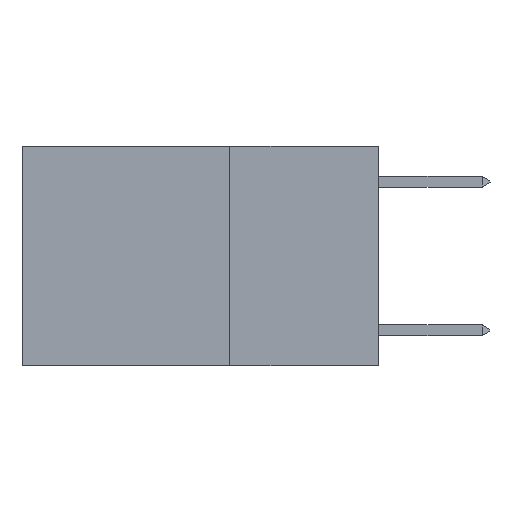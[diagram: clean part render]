
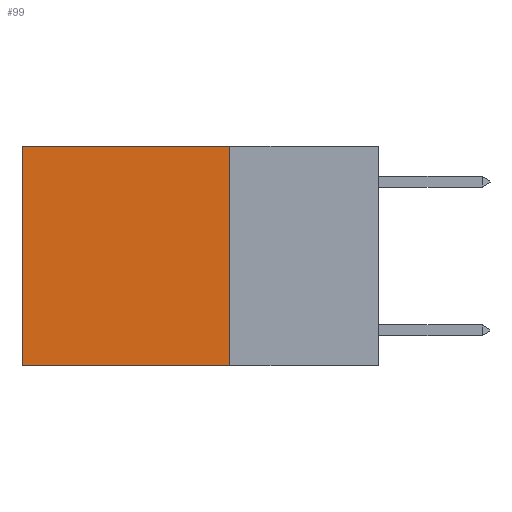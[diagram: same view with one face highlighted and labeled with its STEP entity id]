
A CAD part, left-side view. The second image highlights one B-rep face of the part: STEP entity #99.
In plain terms, the highlighted planar face has unit normal (-1, 0, 0).
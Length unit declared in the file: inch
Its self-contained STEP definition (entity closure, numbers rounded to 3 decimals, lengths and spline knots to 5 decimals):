
#99 = ADVANCED_FACE ( 'NONE', ( #2087 ), #13242, .F. ) ;
#350 = CARTESIAN_POINT ( 'NONE',  ( 0.2625, 0.25, 0. ) ) ;
#652 = CARTESIAN_POINT ( 'NONE',  ( 0.2625, 0.6, -0.37 ) ) ;
#1830 = VECTOR ( 'NONE', #3818, 39.37008 ) ;
#1869 = CARTESIAN_POINT ( 'NONE',  ( 0.2625, 0.6, 0. ) ) ;
#2087 = FACE_OUTER_BOUND ( 'NONE', #12609, .T. ) ;
#2498 = ORIENTED_EDGE ( 'NONE', *, *, #12370, .F. ) ;
#2987 = VERTEX_POINT ( 'NONE', #1869 ) ;
#3550 = CARTESIAN_POINT ( 'NONE',  ( 0.2625, 0.6, 0. ) ) ;
#3818 = DIRECTION ( 'NONE',  ( 0., 1., 0. ) ) ;
#4362 = VERTEX_POINT ( 'NONE', #11102 ) ;
#4703 = DIRECTION ( 'NONE',  ( 0., 1., 0. ) ) ;
#4792 = AXIS2_PLACEMENT_3D ( 'NONE', #12082, #13110, #10972 ) ;
#6037 = DIRECTION ( 'NONE',  ( 0., 0., -1. ) ) ;
#6548 = DIRECTION ( 'NONE',  ( 0., 0., -1. ) ) ;
#7087 = ORIENTED_EDGE ( 'NONE', *, *, #10981, .T. ) ;
#8176 = LINE ( 'NONE', #12398, #11450 ) ;
#8315 = ORIENTED_EDGE ( 'NONE', *, *, #11752, .T. ) ;
#8444 = VECTOR ( 'NONE', #6548, 39.37008 ) ;
#9269 = CARTESIAN_POINT ( 'NONE',  ( 0.2625, 0.25, -0.37 ) ) ;
#9919 = LINE ( 'NONE', #3550, #8444 ) ;
#9956 = CARTESIAN_POINT ( 'NONE',  ( 0.2625, 0.25, -0.37 ) ) ;
#10180 = LINE ( 'NONE', #350, #12650 ) ;
#10280 = LINE ( 'NONE', #9269, #1830 ) ;
#10972 = DIRECTION ( 'NONE',  ( 0., 0., -1. ) ) ;
#10981 = EDGE_CURVE ( 'NONE', #4362, #2987, #10180, .T. ) ;
#11102 = CARTESIAN_POINT ( 'NONE',  ( 0.2625, 0.25, 0. ) ) ;
#11450 = VECTOR ( 'NONE', #6037, 39.37008 ) ;
#11752 = EDGE_CURVE ( 'NONE', #2987, #13862, #9919, .T. ) ;
#11939 = EDGE_CURVE ( 'NONE', #13967, #13862, #10280, .T. ) ;
#12082 = CARTESIAN_POINT ( 'NONE',  ( 0.2625, 0.25, 0. ) ) ;
#12370 = EDGE_CURVE ( 'NONE', #4362, #13967, #8176, .T. ) ;
#12398 = CARTESIAN_POINT ( 'NONE',  ( 0.2625, 0.25, 0. ) ) ;
#12609 = EDGE_LOOP ( 'NONE', ( #8315, #13646, #2498, #7087 ) ) ;
#12650 = VECTOR ( 'NONE', #4703, 39.37008 ) ;
#13110 = DIRECTION ( 'NONE',  ( 1., 0., 0. ) ) ;
#13242 = PLANE ( 'NONE',  #4792 ) ;
#13646 = ORIENTED_EDGE ( 'NONE', *, *, #11939, .F. ) ;
#13862 = VERTEX_POINT ( 'NONE', #652 ) ;
#13967 = VERTEX_POINT ( 'NONE', #9956 ) ;
